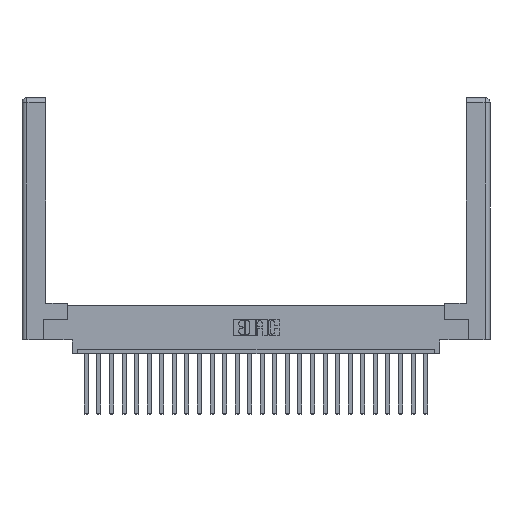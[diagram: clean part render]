
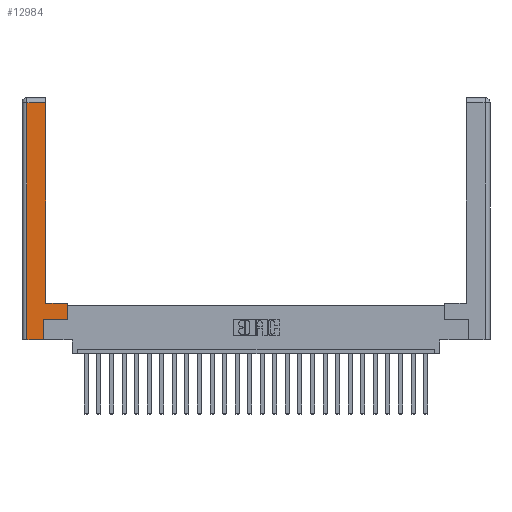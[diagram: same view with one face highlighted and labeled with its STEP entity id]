
A CAD part, top view. The second image highlights one B-rep face of the part: STEP entity #12984.
In plain terms, the highlighted planar face has unit normal (0, 0, 1).
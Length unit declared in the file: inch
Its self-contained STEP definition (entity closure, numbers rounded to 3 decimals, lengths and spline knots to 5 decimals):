
#168 = CARTESIAN_POINT ( 'NONE',  ( 0.265, 0., 0. ) ) ;
#343 = CARTESIAN_POINT ( 'NONE',  ( 0.265, 0.245, 0. ) ) ;
#645 = VECTOR ( 'NONE', #4404, 39.37008 ) ;
#938 = CARTESIAN_POINT ( 'NONE',  ( 0.265, 0., 0. ) ) ;
#1475 = EDGE_CURVE ( 'NONE', #6743, #23452, #21739, .T. ) ;
#1717 = VECTOR ( 'NONE', #5040, 39.37008 ) ;
#1940 = VECTOR ( 'NONE', #8031, 39.37008 ) ;
#2270 = CARTESIAN_POINT ( 'NONE',  ( 0.565, 0.245, 0. ) ) ;
#2335 = LINE ( 'NONE', #19872, #13853 ) ;
#2388 = CARTESIAN_POINT ( 'NONE',  ( 0.565, 0.45, 0. ) ) ;
#2394 = CARTESIAN_POINT ( 'NONE',  ( 0.265, 0.245, 0. ) ) ;
#2453 = EDGE_LOOP ( 'NONE', ( #6864, #20179, #11961, #2914, #18179, #7393, #17687, #10521 ) ) ;
#2778 = EDGE_CURVE ( 'NONE', #14983, #6743, #11005, .T. ) ;
#2914 = ORIENTED_EDGE ( 'NONE', *, *, #10495, .T. ) ;
#3633 = CARTESIAN_POINT ( 'NONE',  ( 0.295, 0.45, 0. ) ) ;
#3781 = DIRECTION ( 'NONE',  ( -1., 0., 0. ) ) ;
#4404 = DIRECTION ( 'NONE',  ( 0., 1., 0. ) ) ;
#5040 = DIRECTION ( 'NONE',  ( 0., -1., 0. ) ) ;
#5344 = VECTOR ( 'NONE', #16391, 39.37008 ) ;
#5680 = CARTESIAN_POINT ( 'NONE',  ( 0.565, 0.45, 0. ) ) ;
#5893 = CARTESIAN_POINT ( 'NONE',  ( 0., 0., 0. ) ) ;
#5956 = VECTOR ( 'NONE', #13484, 39.37008 ) ;
#6027 = FACE_OUTER_BOUND ( 'NONE', #2453, .T. ) ;
#6743 = VERTEX_POINT ( 'NONE', #10849 ) ;
#6864 = ORIENTED_EDGE ( 'NONE', *, *, #19752, .T. ) ;
#7177 = EDGE_CURVE ( 'NONE', #18990, #19295, #10968, .T. ) ;
#7393 = ORIENTED_EDGE ( 'NONE', *, *, #24726, .T. ) ;
#7534 = CARTESIAN_POINT ( 'NONE',  ( 0.0615, 0., 0. ) ) ;
#8031 = DIRECTION ( 'NONE',  ( -1., 0., 0. ) ) ;
#9570 = CARTESIAN_POINT ( 'NONE',  ( 0.0615, 2.94, 0. ) ) ;
#10495 = EDGE_CURVE ( 'NONE', #23452, #18990, #12310, .T. ) ;
#10521 = ORIENTED_EDGE ( 'NONE', *, *, #13780, .T. ) ;
#10849 = CARTESIAN_POINT ( 'NONE',  ( 0.0615, 2.94, 0. ) ) ;
#10968 = LINE ( 'NONE', #2394, #645 ) ;
#11005 = LINE ( 'NONE', #9570, #1940 ) ;
#11307 = LINE ( 'NONE', #21889, #18597 ) ;
#11605 = CARTESIAN_POINT ( 'NONE',  ( 0.565, 0.245, 0. ) ) ;
#11961 = ORIENTED_EDGE ( 'NONE', *, *, #1475, .T. ) ;
#12310 = LINE ( 'NONE', #938, #5344 ) ;
#12984 = ADVANCED_FACE ( 'NONE', ( #6027 ), #17174, .F. ) ;
#13484 = DIRECTION ( 'NONE',  ( 0., 1., 0. ) ) ;
#13780 = EDGE_CURVE ( 'NONE', #17901, #22086, #2335, .T. ) ;
#13853 = VECTOR ( 'NONE', #21990, 39.37008 ) ;
#13990 = CARTESIAN_POINT ( 'NONE',  ( 0.295, 2.94, 0. ) ) ;
#14162 = EDGE_CURVE ( 'NONE', #24227, #17901, #22964, .T. ) ;
#14983 = VERTEX_POINT ( 'NONE', #13990 ) ;
#16391 = DIRECTION ( 'NONE',  ( 1., 0., 0. ) ) ;
#16826 = CARTESIAN_POINT ( 'NONE',  ( 0.0615, 0., 0. ) ) ;
#17174 = PLANE ( 'NONE',  #19652 ) ;
#17473 = DIRECTION ( 'NONE',  ( 1., 0., 0. ) ) ;
#17687 = ORIENTED_EDGE ( 'NONE', *, *, #14162, .T. ) ;
#17901 = VERTEX_POINT ( 'NONE', #2388 ) ;
#17980 = DIRECTION ( 'NONE',  ( 0., 1., 0. ) ) ;
#18179 = ORIENTED_EDGE ( 'NONE', *, *, #7177, .T. ) ;
#18597 = VECTOR ( 'NONE', #17980, 39.37008 ) ;
#18990 = VERTEX_POINT ( 'NONE', #168 ) ;
#19295 = VERTEX_POINT ( 'NONE', #343 ) ;
#19463 = DIRECTION ( 'NONE',  ( 0., 0., -1. ) ) ;
#19652 = AXIS2_PLACEMENT_3D ( 'NONE', #5893, #19463, #3781 ) ;
#19752 = EDGE_CURVE ( 'NONE', #22086, #14983, #11307, .T. ) ;
#19872 = CARTESIAN_POINT ( 'NONE',  ( 0.295, 0.45, 0. ) ) ;
#20179 = ORIENTED_EDGE ( 'NONE', *, *, #2778, .T. ) ;
#21237 = LINE ( 'NONE', #11605, #23079 ) ;
#21739 = LINE ( 'NONE', #16826, #1717 ) ;
#21889 = CARTESIAN_POINT ( 'NONE',  ( 0.295, 3., 0. ) ) ;
#21990 = DIRECTION ( 'NONE',  ( -1., 0., 0. ) ) ;
#22086 = VERTEX_POINT ( 'NONE', #3633 ) ;
#22964 = LINE ( 'NONE', #5680, #5956 ) ;
#23079 = VECTOR ( 'NONE', #17473, 39.37008 ) ;
#23452 = VERTEX_POINT ( 'NONE', #7534 ) ;
#24227 = VERTEX_POINT ( 'NONE', #2270 ) ;
#24726 = EDGE_CURVE ( 'NONE', #19295, #24227, #21237, .T. ) ;
